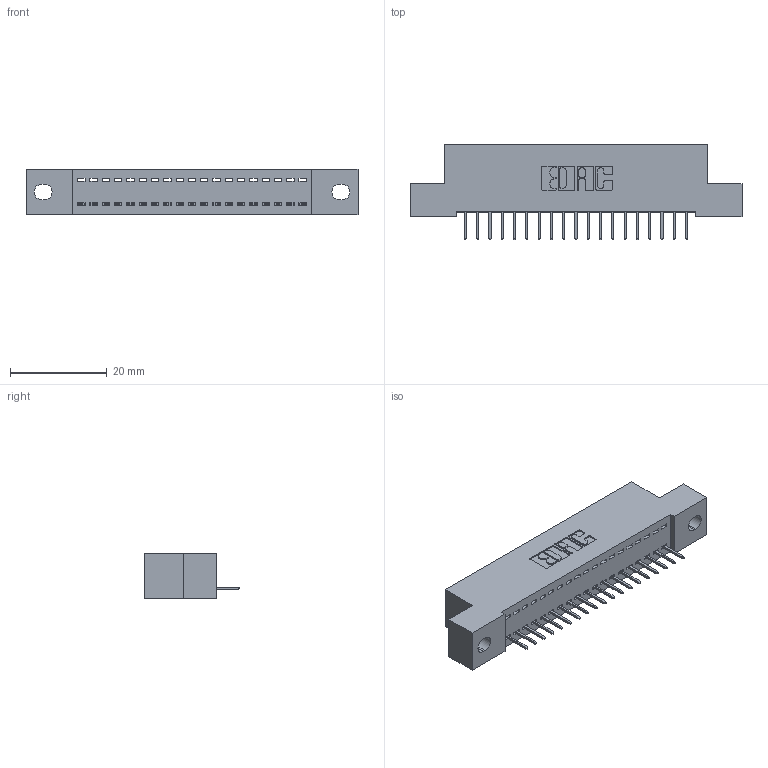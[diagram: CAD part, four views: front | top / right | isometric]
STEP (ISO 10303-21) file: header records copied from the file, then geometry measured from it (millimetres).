
FILE_DESCRIPTION (( 'STEP AP203' ), '1' );
FILE_NAME ('342-019-524-102.STEP', '2019-10-01T20:32:18', ( '' ), ( '' ), 'SwSTEP 2.0', 'SolidWorks 2016', '' );
FILE_SCHEMA (( 'CONFIG_CONTROL_DESIGN' ));
Length unit declared in the file: inch
Products named in the file (3): 342-019-524-102; 342 Part_.128 Slot; 345-292-001_345-293-124
Assembly tree (20 placements, depth 2):
  342-019-524-102
    342 Part_.128 Slot
    345-292-001_345-293-124  x19
Bounding box: 68.58 x 19.69 x 9.4 mm (x, y, z)
Volume: 5801.2 mm3; surface area: 7615.8 mm2
Topology: 20 solids, 20 shells, 1292 faces, 3731 edges, 2410 vertices
Faces by surface type: plane 982, cylinder 310
Entity records: 14667 total; most frequent: CARTESIAN_POINT 2539, ORIENTED_EDGE 2494, DIRECTION 2189, EDGE_CURVE 1247, VECTOR 1123, LINE 1123, VERTEX_POINT 826, AXIS2_PLACEMENT_3D 533
